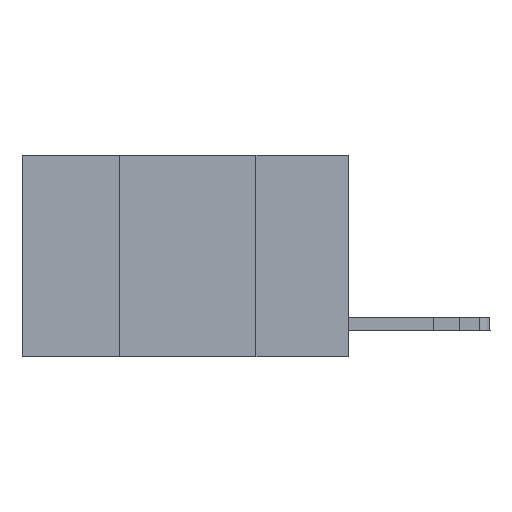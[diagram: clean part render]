
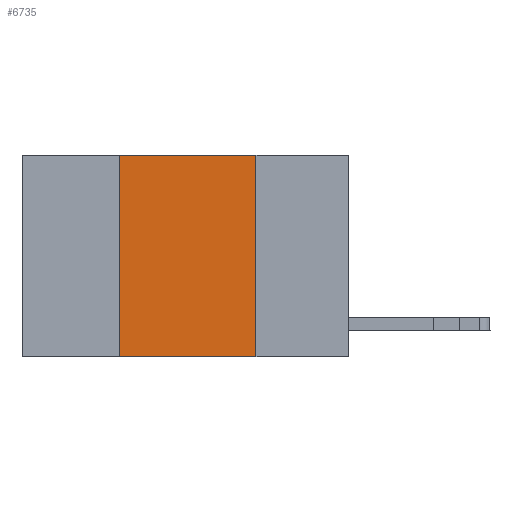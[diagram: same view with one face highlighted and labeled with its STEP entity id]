
A CAD part, left-side view. The second image highlights one B-rep face of the part: STEP entity #6735.
In plain terms, the highlighted planar face has unit normal (-1, 0, 0).
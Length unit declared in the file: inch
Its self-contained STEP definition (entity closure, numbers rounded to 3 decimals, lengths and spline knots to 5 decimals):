
#1316 = VECTOR ( 'NONE', #4788, 39.37008 ) ;
#1492 = EDGE_CURVE ( 'NONE', #8454, #4152, #12983, .T. ) ;
#1610 = CARTESIAN_POINT ( 'NONE',  ( 0., 0.6, 0. ) ) ;
#2961 = VECTOR ( 'NONE', #5627, 39.37008 ) ;
#3075 = LINE ( 'NONE', #10476, #3377 ) ;
#3377 = VECTOR ( 'NONE', #15153, 39.37008 ) ;
#4152 = VERTEX_POINT ( 'NONE', #19249 ) ;
#4416 = CARTESIAN_POINT ( 'NONE',  ( 0., 0.6, 0. ) ) ;
#4788 = DIRECTION ( 'NONE',  ( 0., -1., 0. ) ) ;
#4896 = LINE ( 'NONE', #14296, #1316 ) ;
#5627 = DIRECTION ( 'NONE',  ( 0., 0., -1. ) ) ;
#6054 = CARTESIAN_POINT ( 'NONE',  ( 0., 0.42, -0.37 ) ) ;
#6735 = ADVANCED_FACE ( 'NONE', ( #8060 ), #12278, .F. ) ;
#7599 = LINE ( 'NONE', #4416, #18564 ) ;
#7970 = VERTEX_POINT ( 'NONE', #6054 ) ;
#8060 = FACE_OUTER_BOUND ( 'NONE', #16871, .T. ) ;
#8454 = VERTEX_POINT ( 'NONE', #10549 ) ;
#9502 = DIRECTION ( 'NONE',  ( 0., 0., -1. ) ) ;
#10008 = EDGE_CURVE ( 'NONE', #16060, #8454, #7599, .T. ) ;
#10203 = ORIENTED_EDGE ( 'NONE', *, *, #1492, .F. ) ;
#10373 = DIRECTION ( 'NONE',  ( 0., -1., 0. ) ) ;
#10476 = CARTESIAN_POINT ( 'NONE',  ( 0., 0.42, 0. ) ) ;
#10549 = CARTESIAN_POINT ( 'NONE',  ( 0., 0.17, 0. ) ) ;
#11091 = CARTESIAN_POINT ( 'NONE',  ( 0., 0.42, 0. ) ) ;
#12030 = EDGE_CURVE ( 'NONE', #7970, #4152, #4896, .T. ) ;
#12278 = PLANE ( 'NONE',  #16501 ) ;
#12983 = LINE ( 'NONE', #14512, #2961 ) ;
#14180 = DIRECTION ( 'NONE',  ( 1., 0., 0. ) ) ;
#14296 = CARTESIAN_POINT ( 'NONE',  ( 0., 0.6, -0.37 ) ) ;
#14512 = CARTESIAN_POINT ( 'NONE',  ( 0., 0.17, 0. ) ) ;
#14998 = ORIENTED_EDGE ( 'NONE', *, *, #10008, .F. ) ;
#15153 = DIRECTION ( 'NONE',  ( 0., 0., 1. ) ) ;
#16060 = VERTEX_POINT ( 'NONE', #11091 ) ;
#16501 = AXIS2_PLACEMENT_3D ( 'NONE', #1610, #14180, #9502 ) ;
#16871 = EDGE_LOOP ( 'NONE', ( #10203, #14998, #18885, #18154 ) ) ;
#17208 = EDGE_CURVE ( 'NONE', #7970, #16060, #3075, .T. ) ;
#18154 = ORIENTED_EDGE ( 'NONE', *, *, #12030, .T. ) ;
#18564 = VECTOR ( 'NONE', #10373, 39.37008 ) ;
#18885 = ORIENTED_EDGE ( 'NONE', *, *, #17208, .F. ) ;
#19249 = CARTESIAN_POINT ( 'NONE',  ( 0., 0.17, -0.37 ) ) ;
